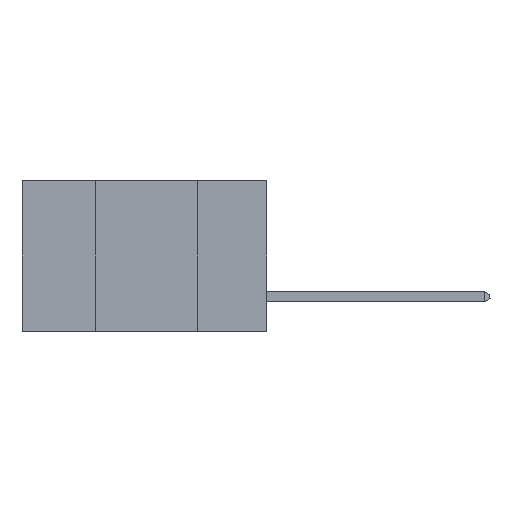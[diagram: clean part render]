
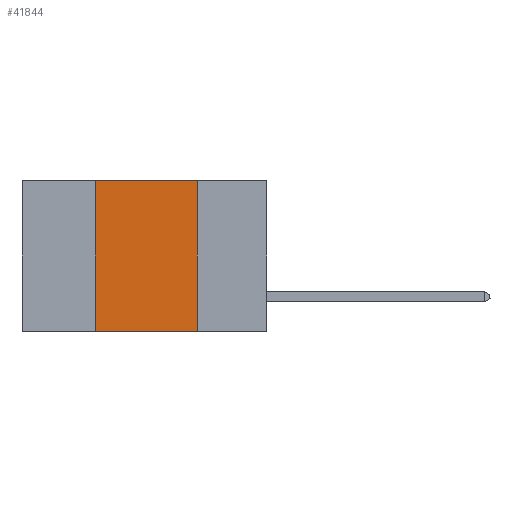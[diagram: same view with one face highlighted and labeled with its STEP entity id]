
A CAD part, left-side view. The second image highlights one B-rep face of the part: STEP entity #41844.
In plain terms, the highlighted planar face has unit normal (-1, 0, 0).
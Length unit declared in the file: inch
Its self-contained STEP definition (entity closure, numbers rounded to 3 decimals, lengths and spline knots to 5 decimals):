
#1488 = DIRECTION ( 'NONE',  ( 0., 0., -1. ) ) ;
#2386 = VECTOR ( 'NONE', #8010, 39.37008 ) ;
#4637 = VERTEX_POINT ( 'NONE', #36132 ) ;
#4696 = CARTESIAN_POINT ( 'NONE',  ( 0., 0.17, 0. ) ) ;
#4823 = CARTESIAN_POINT ( 'NONE',  ( 0., 0.6, 0. ) ) ;
#7172 = LINE ( 'NONE', #32387, #20130 ) ;
#8010 = DIRECTION ( 'NONE',  ( 0., 0., -1. ) ) ;
#9154 = VECTOR ( 'NONE', #35131, 39.37008 ) ;
#9660 = DIRECTION ( 'NONE',  ( 0., -1., 0. ) ) ;
#9840 = ORIENTED_EDGE ( 'NONE', *, *, #31020, .T. ) ;
#10630 = CARTESIAN_POINT ( 'NONE',  ( 0., 0.42, 0. ) ) ;
#12284 = EDGE_CURVE ( 'NONE', #28927, #26963, #18941, .T. ) ;
#12975 = EDGE_LOOP ( 'NONE', ( #35725, #42731, #42602, #9840 ) ) ;
#14824 = VERTEX_POINT ( 'NONE', #24372 ) ;
#18941 = LINE ( 'NONE', #41613, #9154 ) ;
#19931 = FACE_OUTER_BOUND ( 'NONE', #12975, .T. ) ;
#20130 = VECTOR ( 'NONE', #9660, 39.37008 ) ;
#20696 = AXIS2_PLACEMENT_3D ( 'NONE', #4823, #31347, #1488 ) ;
#22020 = LINE ( 'NONE', #4696, #2386 ) ;
#24372 = CARTESIAN_POINT ( 'NONE',  ( 0., 0.42, -0.37 ) ) ;
#24988 = CARTESIAN_POINT ( 'NONE',  ( 0., 0.17, 0. ) ) ;
#26963 = VERTEX_POINT ( 'NONE', #24988 ) ;
#27102 = EDGE_CURVE ( 'NONE', #14824, #28927, #33007, .T. ) ;
#27546 = EDGE_CURVE ( 'NONE', #26963, #4637, #22020, .T. ) ;
#28927 = VERTEX_POINT ( 'NONE', #10630 ) ;
#31020 = EDGE_CURVE ( 'NONE', #14824, #4637, #7172, .T. ) ;
#31347 = DIRECTION ( 'NONE',  ( 1., 0., 0. ) ) ;
#32387 = CARTESIAN_POINT ( 'NONE',  ( 0., 0.6, -0.37 ) ) ;
#33007 = LINE ( 'NONE', #39228, #41754 ) ;
#35131 = DIRECTION ( 'NONE',  ( 0., -1., 0. ) ) ;
#35615 = DIRECTION ( 'NONE',  ( 0., 0., 1. ) ) ;
#35725 = ORIENTED_EDGE ( 'NONE', *, *, #27546, .F. ) ;
#36132 = CARTESIAN_POINT ( 'NONE',  ( 0., 0.17, -0.37 ) ) ;
#39228 = CARTESIAN_POINT ( 'NONE',  ( 0., 0.42, 0. ) ) ;
#40960 = PLANE ( 'NONE',  #20696 ) ;
#41613 = CARTESIAN_POINT ( 'NONE',  ( 0., 0.6, 0. ) ) ;
#41754 = VECTOR ( 'NONE', #35615, 39.37008 ) ;
#41844 = ADVANCED_FACE ( 'NONE', ( #19931 ), #40960, .F. ) ;
#42602 = ORIENTED_EDGE ( 'NONE', *, *, #27102, .F. ) ;
#42731 = ORIENTED_EDGE ( 'NONE', *, *, #12284, .F. ) ;
